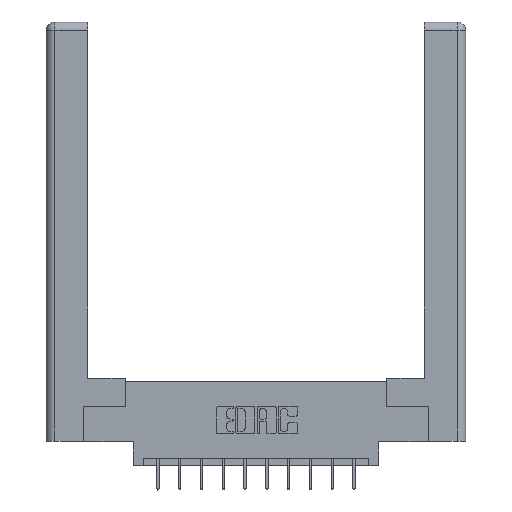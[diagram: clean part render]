
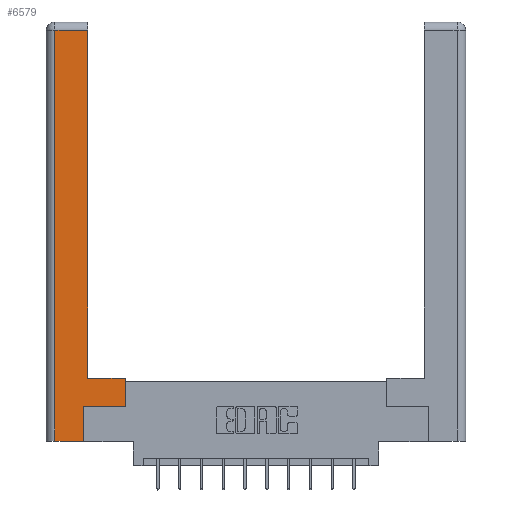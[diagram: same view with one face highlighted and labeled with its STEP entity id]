
A CAD part, top view. The second image highlights one B-rep face of the part: STEP entity #6579.
In plain terms, the highlighted planar face has unit normal (0, 0, 1).
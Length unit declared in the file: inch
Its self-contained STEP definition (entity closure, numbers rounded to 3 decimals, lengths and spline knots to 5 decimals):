
#3 = VERTEX_POINT ( 'NONE', #13872 ) ;
#527 = VECTOR ( 'NONE', #12075, 39.37008 ) ;
#673 = ORIENTED_EDGE ( 'NONE', *, *, #2200, .T. ) ;
#697 = LINE ( 'NONE', #8643, #9257 ) ;
#1488 = DIRECTION ( 'NONE',  ( 1., 0., 0. ) ) ;
#1598 = EDGE_CURVE ( 'NONE', #3, #12074, #9618, .T. ) ;
#1846 = VERTEX_POINT ( 'NONE', #6103 ) ;
#1906 = DIRECTION ( 'NONE',  ( -1., 0., 0. ) ) ;
#1959 = EDGE_CURVE ( 'NONE', #3357, #8360, #11400, .T. ) ;
#2178 = LINE ( 'NONE', #5415, #9678 ) ;
#2199 = CARTESIAN_POINT ( 'NONE',  ( 0.265, 0.245, 0. ) ) ;
#2200 = EDGE_CURVE ( 'NONE', #10367, #1846, #6029, .T. ) ;
#2248 = VECTOR ( 'NONE', #12114, 39.37008 ) ;
#2927 = EDGE_CURVE ( 'NONE', #12074, #3357, #697, .T. ) ;
#3347 = ORIENTED_EDGE ( 'NONE', *, *, #1959, .T. ) ;
#3357 = VERTEX_POINT ( 'NONE', #11869 ) ;
#3423 = VERTEX_POINT ( 'NONE', #7444 ) ;
#3975 = CARTESIAN_POINT ( 'NONE',  ( 0.0615, 2.94, 0. ) ) ;
#4113 = PLANE ( 'NONE',  #9762 ) ;
#4209 = EDGE_CURVE ( 'NONE', #8360, #12227, #9036, .T. ) ;
#5005 = LINE ( 'NONE', #10936, #527 ) ;
#5070 = DIRECTION ( 'NONE',  ( -1., 0., 0. ) ) ;
#5261 = DIRECTION ( 'NONE',  ( 0., 0., -1. ) ) ;
#5415 = CARTESIAN_POINT ( 'NONE',  ( 0.565, 0.45, 0. ) ) ;
#5865 = VECTOR ( 'NONE', #5070, 39.37008 ) ;
#5901 = DIRECTION ( 'NONE',  ( 1., 0., 0. ) ) ;
#6029 = LINE ( 'NONE', #7292, #7989 ) ;
#6103 = CARTESIAN_POINT ( 'NONE',  ( 0.565, 0.245, 0. ) ) ;
#6408 = CARTESIAN_POINT ( 'NONE',  ( 0.295, 0.45, 0. ) ) ;
#6579 = ADVANCED_FACE ( 'NONE', ( #14470 ), #4113, .F. ) ;
#6690 = EDGE_CURVE ( 'NONE', #1846, #3, #2178, .T. ) ;
#7292 = CARTESIAN_POINT ( 'NONE',  ( 0.565, 0.245, 0. ) ) ;
#7444 = CARTESIAN_POINT ( 'NONE',  ( 0.265, 0., 0. ) ) ;
#7503 = CARTESIAN_POINT ( 'NONE',  ( 0.0615, 2.94, 0. ) ) ;
#7834 = VECTOR ( 'NONE', #13260, 39.37008 ) ;
#7989 = VECTOR ( 'NONE', #1488, 39.37008 ) ;
#8360 = VERTEX_POINT ( 'NONE', #7503 ) ;
#8363 = EDGE_CURVE ( 'NONE', #3423, #10367, #5005, .T. ) ;
#8643 = CARTESIAN_POINT ( 'NONE',  ( 0.295, 3., 0. ) ) ;
#9036 = LINE ( 'NONE', #12165, #2248 ) ;
#9048 = CARTESIAN_POINT ( 'NONE',  ( 0.0615, 0., 0. ) ) ;
#9257 = VECTOR ( 'NONE', #12081, 39.37008 ) ;
#9470 = ORIENTED_EDGE ( 'NONE', *, *, #10037, .T. ) ;
#9598 = ORIENTED_EDGE ( 'NONE', *, *, #4209, .T. ) ;
#9618 = LINE ( 'NONE', #6408, #7834 ) ;
#9678 = VECTOR ( 'NONE', #10046, 39.37008 ) ;
#9762 = AXIS2_PLACEMENT_3D ( 'NONE', #11981, #5261, #1906 ) ;
#10037 = EDGE_CURVE ( 'NONE', #12227, #3423, #14109, .T. ) ;
#10046 = DIRECTION ( 'NONE',  ( 0., 1., 0. ) ) ;
#10277 = ORIENTED_EDGE ( 'NONE', *, *, #2927, .T. ) ;
#10367 = VERTEX_POINT ( 'NONE', #2199 ) ;
#10443 = CARTESIAN_POINT ( 'NONE',  ( 0.265, 0., 0. ) ) ;
#10936 = CARTESIAN_POINT ( 'NONE',  ( 0.265, 0.245, 0. ) ) ;
#11105 = VECTOR ( 'NONE', #5901, 39.37008 ) ;
#11266 = ORIENTED_EDGE ( 'NONE', *, *, #8363, .T. ) ;
#11400 = LINE ( 'NONE', #3975, #5865 ) ;
#11869 = CARTESIAN_POINT ( 'NONE',  ( 0.295, 2.94, 0. ) ) ;
#11981 = CARTESIAN_POINT ( 'NONE',  ( 0., 0., 0. ) ) ;
#12044 = ORIENTED_EDGE ( 'NONE', *, *, #1598, .T. ) ;
#12074 = VERTEX_POINT ( 'NONE', #13164 ) ;
#12075 = DIRECTION ( 'NONE',  ( 0., 1., 0. ) ) ;
#12081 = DIRECTION ( 'NONE',  ( 0., 1., 0. ) ) ;
#12114 = DIRECTION ( 'NONE',  ( 0., -1., 0. ) ) ;
#12165 = CARTESIAN_POINT ( 'NONE',  ( 0.0615, 0., 0. ) ) ;
#12227 = VERTEX_POINT ( 'NONE', #9048 ) ;
#13164 = CARTESIAN_POINT ( 'NONE',  ( 0.295, 0.45, 0. ) ) ;
#13260 = DIRECTION ( 'NONE',  ( -1., 0., 0. ) ) ;
#13872 = CARTESIAN_POINT ( 'NONE',  ( 0.565, 0.45, 0. ) ) ;
#14069 = EDGE_LOOP ( 'NONE', ( #10277, #3347, #9598, #9470, #11266, #673, #14679, #12044 ) ) ;
#14109 = LINE ( 'NONE', #10443, #11105 ) ;
#14470 = FACE_OUTER_BOUND ( 'NONE', #14069, .T. ) ;
#14679 = ORIENTED_EDGE ( 'NONE', *, *, #6690, .T. ) ;
